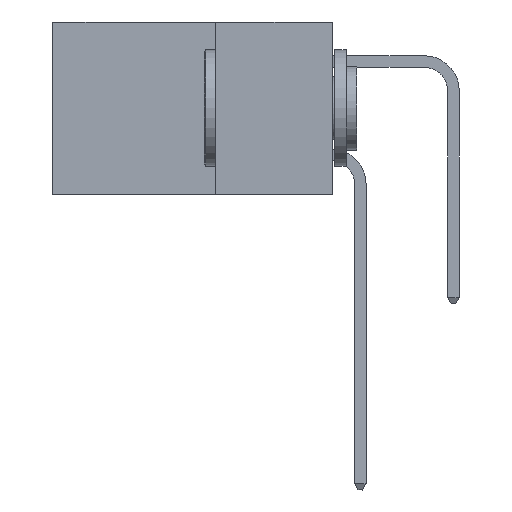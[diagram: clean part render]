
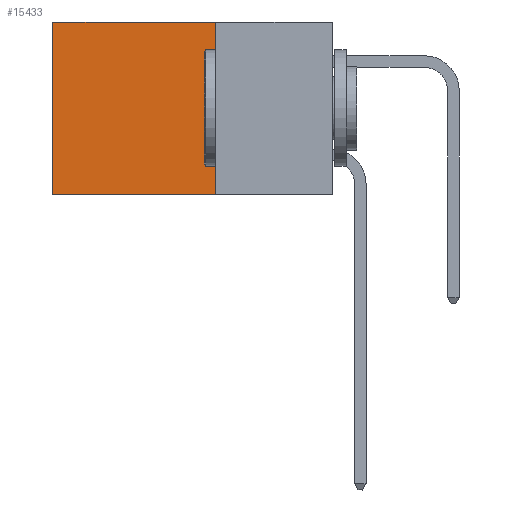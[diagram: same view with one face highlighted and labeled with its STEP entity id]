
A CAD part, left-side view. The second image highlights one B-rep face of the part: STEP entity #15433.
In plain terms, the highlighted planar face has unit normal (-1, 0, 0).
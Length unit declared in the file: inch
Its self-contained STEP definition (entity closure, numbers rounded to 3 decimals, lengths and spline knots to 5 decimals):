
#366 = VERTEX_POINT ( 'NONE', #4087 ) ;
#1461 = CARTESIAN_POINT ( 'NONE',  ( 0.298, 0.6, 0. ) ) ;
#1684 = ORIENTED_EDGE ( 'NONE', *, *, #14730, .F. ) ;
#3109 = EDGE_CURVE ( 'NONE', #366, #15611, #15101, .T. ) ;
#3828 = ORIENTED_EDGE ( 'NONE', *, *, #4922, .F. ) ;
#3950 = DIRECTION ( 'NONE',  ( 0., 0., -1. ) ) ;
#4087 = CARTESIAN_POINT ( 'NONE',  ( 0.298, 0.25, 0. ) ) ;
#4651 = VECTOR ( 'NONE', #3950, 39.37008 ) ;
#4690 = VECTOR ( 'NONE', #10114, 39.37008 ) ;
#4922 = EDGE_CURVE ( 'NONE', #366, #7324, #12525, .T. ) ;
#6617 = CARTESIAN_POINT ( 'NONE',  ( 0.298, 0.6, -0.37 ) ) ;
#6902 = ORIENTED_EDGE ( 'NONE', *, *, #12747, .T. ) ;
#7316 = CARTESIAN_POINT ( 'NONE',  ( 0.298, 0.25, 0. ) ) ;
#7324 = VERTEX_POINT ( 'NONE', #15878 ) ;
#8167 = LINE ( 'NONE', #1461, #15294 ) ;
#8745 = LINE ( 'NONE', #12911, #4690 ) ;
#8754 = DIRECTION ( 'NONE',  ( 0., 0., -1. ) ) ;
#9431 = VERTEX_POINT ( 'NONE', #6617 ) ;
#9880 = DIRECTION ( 'NONE',  ( 0., 0., -1. ) ) ;
#10114 = DIRECTION ( 'NONE',  ( 0., 1., 0. ) ) ;
#10134 = EDGE_LOOP ( 'NONE', ( #6902, #1684, #3828, #17639 ) ) ;
#10905 = VECTOR ( 'NONE', #14756, 39.37008 ) ;
#11574 = PLANE ( 'NONE',  #12884 ) ;
#12525 = LINE ( 'NONE', #16465, #4651 ) ;
#12747 = EDGE_CURVE ( 'NONE', #15611, #9431, #8167, .T. ) ;
#12884 = AXIS2_PLACEMENT_3D ( 'NONE', #7316, #17212, #8754 ) ;
#12911 = CARTESIAN_POINT ( 'NONE',  ( 0.298, 0.25, -0.37 ) ) ;
#14730 = EDGE_CURVE ( 'NONE', #7324, #9431, #8745, .T. ) ;
#14756 = DIRECTION ( 'NONE',  ( 0., 1., 0. ) ) ;
#14789 = CARTESIAN_POINT ( 'NONE',  ( 0.298, 0.6, 0. ) ) ;
#15101 = LINE ( 'NONE', #16349, #10905 ) ;
#15185 = FACE_OUTER_BOUND ( 'NONE', #10134, .T. ) ;
#15294 = VECTOR ( 'NONE', #9880, 39.37008 ) ;
#15433 = ADVANCED_FACE ( 'NONE', ( #15185 ), #11574, .F. ) ;
#15611 = VERTEX_POINT ( 'NONE', #14789 ) ;
#15878 = CARTESIAN_POINT ( 'NONE',  ( 0.298, 0.25, -0.37 ) ) ;
#16349 = CARTESIAN_POINT ( 'NONE',  ( 0.298, 0.25, 0. ) ) ;
#16465 = CARTESIAN_POINT ( 'NONE',  ( 0.298, 0.25, 0. ) ) ;
#17212 = DIRECTION ( 'NONE',  ( 1., 0., 0. ) ) ;
#17639 = ORIENTED_EDGE ( 'NONE', *, *, #3109, .T. ) ;
